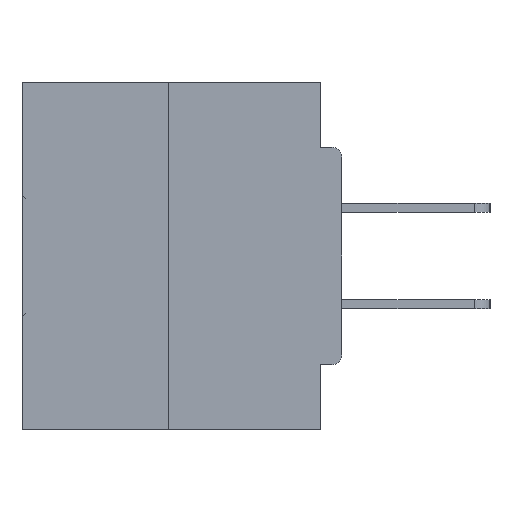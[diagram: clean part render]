
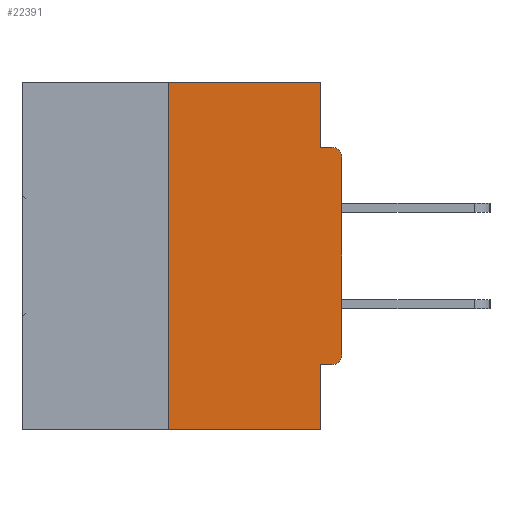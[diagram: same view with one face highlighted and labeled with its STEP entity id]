
A CAD part, left-side view. The second image highlights one B-rep face of the part: STEP entity #22391.
In plain terms, the highlighted planar face has unit normal (-1, 0, 0).
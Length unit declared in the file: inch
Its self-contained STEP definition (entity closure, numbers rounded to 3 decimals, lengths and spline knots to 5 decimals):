
#28 = CARTESIAN_POINT ( 'NONE',  ( 0., 0.031, -0.4065 ) ) ;
#1406 = VERTEX_POINT ( 'NONE', #13008 ) ;
#1455 = VERTEX_POINT ( 'NONE', #16092 ) ;
#1820 = DIRECTION ( 'NONE',  ( 0., 0., -1. ) ) ;
#3906 = CARTESIAN_POINT ( 'NONE',  ( 0., 0.25, -0.5 ) ) ;
#4016 = EDGE_CURVE ( 'NONE', #19762, #21160, #18945, .T. ) ;
#4456 = LINE ( 'NONE', #7447, #33489 ) ;
#4929 = VECTOR ( 'NONE', #22880, 39.37008 ) ;
#4964 = CARTESIAN_POINT ( 'NONE',  ( 0., 0.031, -0.5 ) ) ;
#5311 = AXIS2_PLACEMENT_3D ( 'NONE', #42819, #32878, #16220 ) ;
#5550 = VECTOR ( 'NONE', #33527, 39.37008 ) ;
#7356 = VERTEX_POINT ( 'NONE', #28 ) ;
#7447 = CARTESIAN_POINT ( 'NONE',  ( 0., 0.25, 0. ) ) ;
#7736 = FACE_OUTER_BOUND ( 'NONE', #32088, .T. ) ;
#7815 = DIRECTION ( 'NONE',  ( 0., -1., 0. ) ) ;
#8415 = CARTESIAN_POINT ( 'NONE',  ( 0., 0.031, -0.5 ) ) ;
#10597 = DIRECTION ( 'NONE',  ( 0., 0., -1. ) ) ;
#10828 = EDGE_CURVE ( 'NONE', #16792, #24253, #39511, .T. ) ;
#11304 = VERTEX_POINT ( 'NONE', #42645 ) ;
#11463 = DIRECTION ( 'NONE',  ( -1., 0., 0. ) ) ;
#11824 = PLANE ( 'NONE',  #28056 ) ;
#12212 = CARTESIAN_POINT ( 'NONE',  ( 0., 0.031, 0. ) ) ;
#12905 = AXIS2_PLACEMENT_3D ( 'NONE', #31673, #11463, #14851 ) ;
#13008 = CARTESIAN_POINT ( 'NONE',  ( 0., 0.015, -0.4065 ) ) ;
#13938 = LINE ( 'NONE', #32911, #4929 ) ;
#13981 = EDGE_CURVE ( 'NONE', #1406, #7356, #28243, .T. ) ;
#14057 = EDGE_CURVE ( 'NONE', #19762, #32599, #4456, .T. ) ;
#14825 = ORIENTED_EDGE ( 'NONE', *, *, #30378, .T. ) ;
#14851 = DIRECTION ( 'NONE',  ( 0., 0., -1. ) ) ;
#15304 = EDGE_CURVE ( 'NONE', #32599, #20062, #13938, .T. ) ;
#15625 = LINE ( 'NONE', #4964, #30424 ) ;
#16092 = CARTESIAN_POINT ( 'NONE',  ( 0., 0., -0.1085 ) ) ;
#16220 = DIRECTION ( 'NONE',  ( 0., 0., -1. ) ) ;
#16722 = VECTOR ( 'NONE', #10597, 39.37008 ) ;
#16792 = VERTEX_POINT ( 'NONE', #39515 ) ;
#17057 = CARTESIAN_POINT ( 'NONE',  ( 0., 0., -0.4065 ) ) ;
#17166 = DIRECTION ( 'NONE',  ( 0., 0., 1. ) ) ;
#18060 = DIRECTION ( 'NONE',  ( 1., 0., 0. ) ) ;
#18544 = DIRECTION ( 'NONE',  ( 0., 0., 1. ) ) ;
#18945 = LINE ( 'NONE', #34010, #30570 ) ;
#19371 = EDGE_CURVE ( 'NONE', #7356, #21160, #15625, .T. ) ;
#19762 = VERTEX_POINT ( 'NONE', #3906 ) ;
#20062 = VERTEX_POINT ( 'NONE', #37581 ) ;
#20426 = EDGE_CURVE ( 'NONE', #11304, #1455, #29996, .T. ) ;
#21160 = VERTEX_POINT ( 'NONE', #8415 ) ;
#21228 = EDGE_CURVE ( 'NONE', #20062, #16792, #25761, .T. ) ;
#21640 = ORIENTED_EDGE ( 'NONE', *, *, #20426, .T. ) ;
#22391 = ADVANCED_FACE ( 'NONE', ( #7736 ), #11824, .F. ) ;
#22880 = DIRECTION ( 'NONE',  ( 0., -1., 0. ) ) ;
#23327 = ORIENTED_EDGE ( 'NONE', *, *, #13981, .F. ) ;
#24253 = VERTEX_POINT ( 'NONE', #41252 ) ;
#24984 = ORIENTED_EDGE ( 'NONE', *, *, #14057, .F. ) ;
#25761 = LINE ( 'NONE', #12212, #16722 ) ;
#25869 = ORIENTED_EDGE ( 'NONE', *, *, #10828, .F. ) ;
#26058 = ORIENTED_EDGE ( 'NONE', *, *, #21228, .F. ) ;
#26744 = EDGE_CURVE ( 'NONE', #1406, #11304, #28938, .T. ) ;
#27358 = CARTESIAN_POINT ( 'NONE',  ( 0., 0.25, 0. ) ) ;
#28056 = AXIS2_PLACEMENT_3D ( 'NONE', #35433, #18060, #28245 ) ;
#28243 = LINE ( 'NONE', #17057, #5550 ) ;
#28245 = DIRECTION ( 'NONE',  ( 0., 0., -1. ) ) ;
#28938 = CIRCLE ( 'NONE', #12905, 0.015 ) ;
#29563 = VECTOR ( 'NONE', #7815, 39.37008 ) ;
#29666 = CIRCLE ( 'NONE', #5311, 0.015 ) ;
#29996 = LINE ( 'NONE', #38983, #35286 ) ;
#30378 = EDGE_CURVE ( 'NONE', #1455, #24253, #29666, .T. ) ;
#30424 = VECTOR ( 'NONE', #1820, 39.37008 ) ;
#30570 = VECTOR ( 'NONE', #34296, 39.37008 ) ;
#31093 = ORIENTED_EDGE ( 'NONE', *, *, #26744, .T. ) ;
#31673 = CARTESIAN_POINT ( 'NONE',  ( 0., 0.015, -0.3915 ) ) ;
#32088 = EDGE_LOOP ( 'NONE', ( #36851, #24984, #32435, #34656, #23327, #31093, #21640, #14825, #25869, #26058 ) ) ;
#32435 = ORIENTED_EDGE ( 'NONE', *, *, #4016, .T. ) ;
#32599 = VERTEX_POINT ( 'NONE', #27358 ) ;
#32878 = DIRECTION ( 'NONE',  ( -1., 0., 0. ) ) ;
#32911 = CARTESIAN_POINT ( 'NONE',  ( 0., 0.46, 0. ) ) ;
#33489 = VECTOR ( 'NONE', #17166, 39.37008 ) ;
#33527 = DIRECTION ( 'NONE',  ( 0., 1., 0. ) ) ;
#34010 = CARTESIAN_POINT ( 'NONE',  ( 0., 0.46, -0.5 ) ) ;
#34296 = DIRECTION ( 'NONE',  ( 0., -1., 0. ) ) ;
#34503 = CARTESIAN_POINT ( 'NONE',  ( 0., 0., -0.0935 ) ) ;
#34656 = ORIENTED_EDGE ( 'NONE', *, *, #19371, .F. ) ;
#35286 = VECTOR ( 'NONE', #18544, 39.37008 ) ;
#35433 = CARTESIAN_POINT ( 'NONE',  ( 0., 0.46, 0. ) ) ;
#36851 = ORIENTED_EDGE ( 'NONE', *, *, #15304, .F. ) ;
#37581 = CARTESIAN_POINT ( 'NONE',  ( 0., 0.031, 0. ) ) ;
#38983 = CARTESIAN_POINT ( 'NONE',  ( 0., 0., 0. ) ) ;
#39511 = LINE ( 'NONE', #34503, #29563 ) ;
#39515 = CARTESIAN_POINT ( 'NONE',  ( 0., 0.031, -0.0935 ) ) ;
#41252 = CARTESIAN_POINT ( 'NONE',  ( 0., 0.015, -0.0935 ) ) ;
#42645 = CARTESIAN_POINT ( 'NONE',  ( 0., 0., -0.3915 ) ) ;
#42819 = CARTESIAN_POINT ( 'NONE',  ( 0., 0.015, -0.1085 ) ) ;
